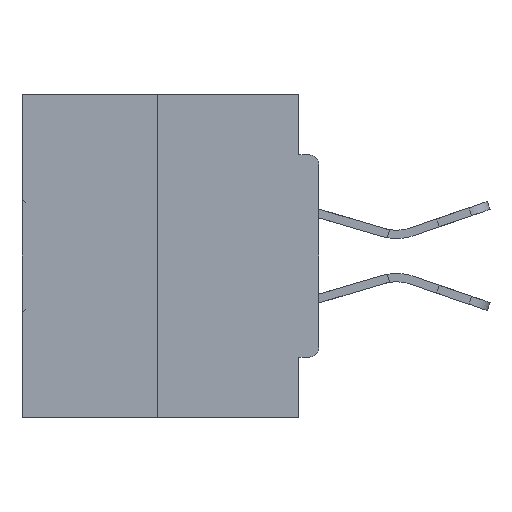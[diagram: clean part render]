
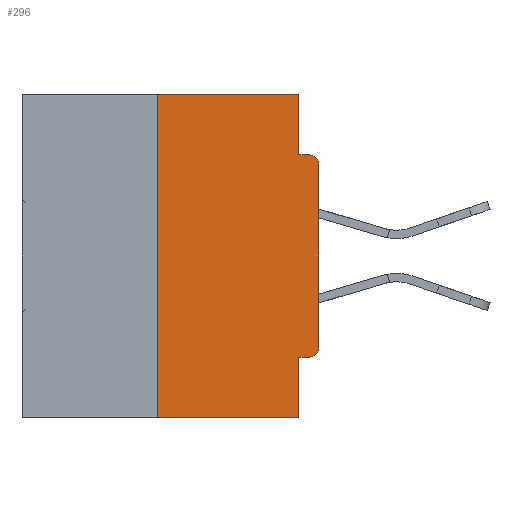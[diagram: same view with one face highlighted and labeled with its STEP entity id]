
A CAD part, left-side view. The second image highlights one B-rep face of the part: STEP entity #296.
In plain terms, the highlighted planar face has unit normal (-1, 0, 0).
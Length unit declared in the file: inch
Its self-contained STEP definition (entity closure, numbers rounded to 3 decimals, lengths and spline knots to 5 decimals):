
#296 = ADVANCED_FACE ( 'NONE', ( #27219 ), #1460, .F. ) ;
#494 = EDGE_CURVE ( 'NONE', #9583, #31604, #43213, .T. ) ;
#1460 = PLANE ( 'NONE',  #32072 ) ;
#1561 = VECTOR ( 'NONE', #42959, 39.37008 ) ;
#2095 = CIRCLE ( 'NONE', #25626, 0.015 ) ;
#2530 = EDGE_CURVE ( 'NONE', #31604, #31346, #6596, .T. ) ;
#2940 = VERTEX_POINT ( 'NONE', #24029 ) ;
#3154 = ORIENTED_EDGE ( 'NONE', *, *, #9521, .F. ) ;
#3176 = DIRECTION ( 'NONE',  ( 0., -1., 0. ) ) ;
#3772 = CARTESIAN_POINT ( 'NONE',  ( 0., 0., -0.4065 ) ) ;
#3836 = CARTESIAN_POINT ( 'NONE',  ( 0., 0., 0. ) ) ;
#3909 = EDGE_CURVE ( 'NONE', #23401, #31346, #6555, .T. ) ;
#4751 = VECTOR ( 'NONE', #21584, 39.37008 ) ;
#5307 = CARTESIAN_POINT ( 'NONE',  ( 0., 0.031, -0.0935 ) ) ;
#5498 = VECTOR ( 'NONE', #17285, 39.37008 ) ;
#6555 = CIRCLE ( 'NONE', #43601, 0.015 ) ;
#6596 = LINE ( 'NONE', #40622, #14928 ) ;
#7778 = VERTEX_POINT ( 'NONE', #13528 ) ;
#7828 = CARTESIAN_POINT ( 'NONE',  ( 0., 0.031, 0. ) ) ;
#7870 = EDGE_CURVE ( 'NONE', #34426, #9583, #21477, .T. ) ;
#8828 = ORIENTED_EDGE ( 'NONE', *, *, #7870, .F. ) ;
#9349 = CARTESIAN_POINT ( 'NONE',  ( 0., 0.46, -0.5 ) ) ;
#9521 = EDGE_CURVE ( 'NONE', #2940, #34426, #20744, .T. ) ;
#9583 = VERTEX_POINT ( 'NONE', #7828 ) ;
#10889 = LINE ( 'NONE', #18244, #1561 ) ;
#10943 = CARTESIAN_POINT ( 'NONE',  ( 0., 0., -0.3915 ) ) ;
#11088 = VECTOR ( 'NONE', #3176, 39.37008 ) ;
#13528 = CARTESIAN_POINT ( 'NONE',  ( 0., 0.031, -0.4065 ) ) ;
#14044 = CARTESIAN_POINT ( 'NONE',  ( 0., 0.015, -0.0935 ) ) ;
#14354 = CARTESIAN_POINT ( 'NONE',  ( 0., 0.015, -0.1085 ) ) ;
#14494 = DIRECTION ( 'NONE',  ( 0., 0., 1. ) ) ;
#14499 = EDGE_LOOP ( 'NONE', ( #8828, #3154, #43666, #43263, #18918, #42453, #28081, #21114, #41621, #29087 ) ) ;
#14928 = VECTOR ( 'NONE', #44132, 39.37008 ) ;
#16421 = CARTESIAN_POINT ( 'NONE',  ( 0., 0., -0.1085 ) ) ;
#17285 = DIRECTION ( 'NONE',  ( 0., -1., 0. ) ) ;
#17558 = CARTESIAN_POINT ( 'NONE',  ( 0., 0.25, 0. ) ) ;
#18244 = CARTESIAN_POINT ( 'NONE',  ( 0., 0.031, -0.5 ) ) ;
#18918 = ORIENTED_EDGE ( 'NONE', *, *, #31425, .F. ) ;
#20374 = DIRECTION ( 'NONE',  ( -1., 0., 0. ) ) ;
#20744 = LINE ( 'NONE', #17558, #4751 ) ;
#21114 = ORIENTED_EDGE ( 'NONE', *, *, #3909, .T. ) ;
#21477 = LINE ( 'NONE', #35132, #5498 ) ;
#21584 = DIRECTION ( 'NONE',  ( 0., 0., 1. ) ) ;
#21673 = DIRECTION ( 'NONE',  ( 0., 1., 0. ) ) ;
#21753 = DIRECTION ( 'NONE',  ( -1., 0., 0. ) ) ;
#22636 = EDGE_CURVE ( 'NONE', #34101, #34933, #2095, .T. ) ;
#23401 = VERTEX_POINT ( 'NONE', #16421 ) ;
#24029 = CARTESIAN_POINT ( 'NONE',  ( 0., 0.25, -0.5 ) ) ;
#25294 = DIRECTION ( 'NONE',  ( 0., 0., -1. ) ) ;
#25626 = AXIS2_PLACEMENT_3D ( 'NONE', #34667, #20374, #27700 ) ;
#25705 = LINE ( 'NONE', #3836, #41085 ) ;
#26359 = DIRECTION ( 'NONE',  ( 1., 0., 0. ) ) ;
#27219 = FACE_OUTER_BOUND ( 'NONE', #14499, .T. ) ;
#27700 = DIRECTION ( 'NONE',  ( 0., 0., -1. ) ) ;
#28081 = ORIENTED_EDGE ( 'NONE', *, *, #33153, .T. ) ;
#28353 = CARTESIAN_POINT ( 'NONE',  ( 0., 0.031, 0. ) ) ;
#29087 = ORIENTED_EDGE ( 'NONE', *, *, #494, .F. ) ;
#30947 = CARTESIAN_POINT ( 'NONE',  ( 0., 0.015, -0.4065 ) ) ;
#31299 = VECTOR ( 'NONE', #21673, 39.37008 ) ;
#31346 = VERTEX_POINT ( 'NONE', #14044 ) ;
#31425 = EDGE_CURVE ( 'NONE', #34101, #7778, #42861, .T. ) ;
#31604 = VERTEX_POINT ( 'NONE', #5307 ) ;
#31902 = EDGE_CURVE ( 'NONE', #7778, #34081, #10889, .T. ) ;
#32072 = AXIS2_PLACEMENT_3D ( 'NONE', #36705, #26359, #33642 ) ;
#33153 = EDGE_CURVE ( 'NONE', #34933, #23401, #25705, .T. ) ;
#33642 = DIRECTION ( 'NONE',  ( 0., 0., -1. ) ) ;
#34081 = VERTEX_POINT ( 'NONE', #38444 ) ;
#34101 = VERTEX_POINT ( 'NONE', #30947 ) ;
#34426 = VERTEX_POINT ( 'NONE', #38177 ) ;
#34667 = CARTESIAN_POINT ( 'NONE',  ( 0., 0.015, -0.3915 ) ) ;
#34767 = LINE ( 'NONE', #9349, #11088 ) ;
#34933 = VERTEX_POINT ( 'NONE', #10943 ) ;
#34960 = VECTOR ( 'NONE', #42033, 39.37008 ) ;
#35132 = CARTESIAN_POINT ( 'NONE',  ( 0., 0.46, 0. ) ) ;
#36705 = CARTESIAN_POINT ( 'NONE',  ( 0., 0.46, 0. ) ) ;
#38177 = CARTESIAN_POINT ( 'NONE',  ( 0., 0.25, 0. ) ) ;
#38444 = CARTESIAN_POINT ( 'NONE',  ( 0., 0.031, -0.5 ) ) ;
#38979 = EDGE_CURVE ( 'NONE', #2940, #34081, #34767, .T. ) ;
#40622 = CARTESIAN_POINT ( 'NONE',  ( 0., 0., -0.0935 ) ) ;
#41085 = VECTOR ( 'NONE', #14494, 39.37008 ) ;
#41621 = ORIENTED_EDGE ( 'NONE', *, *, #2530, .F. ) ;
#42033 = DIRECTION ( 'NONE',  ( 0., 0., -1. ) ) ;
#42453 = ORIENTED_EDGE ( 'NONE', *, *, #22636, .T. ) ;
#42861 = LINE ( 'NONE', #3772, #31299 ) ;
#42959 = DIRECTION ( 'NONE',  ( 0., 0., -1. ) ) ;
#43213 = LINE ( 'NONE', #28353, #34960 ) ;
#43263 = ORIENTED_EDGE ( 'NONE', *, *, #31902, .F. ) ;
#43601 = AXIS2_PLACEMENT_3D ( 'NONE', #14354, #21753, #25294 ) ;
#43666 = ORIENTED_EDGE ( 'NONE', *, *, #38979, .T. ) ;
#44132 = DIRECTION ( 'NONE',  ( 0., -1., 0. ) ) ;
